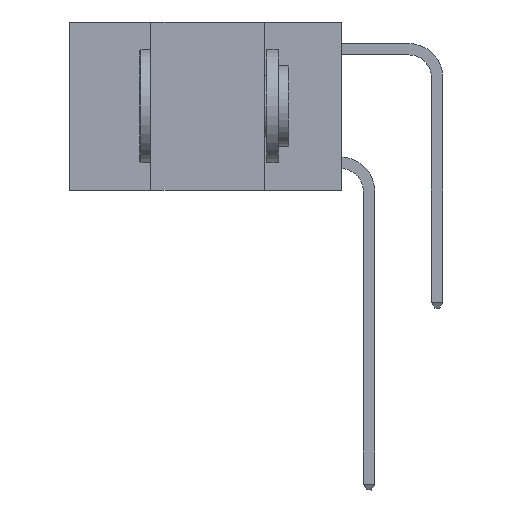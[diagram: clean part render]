
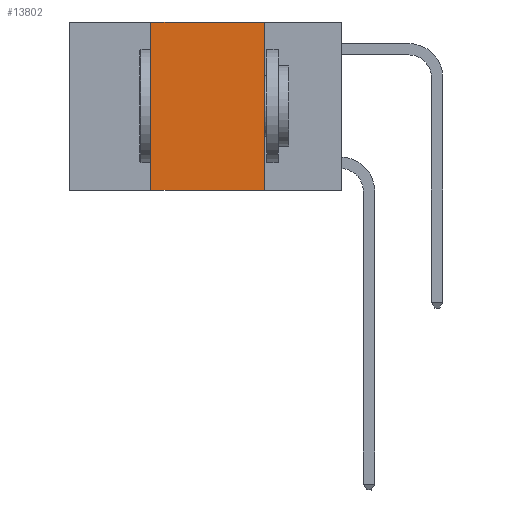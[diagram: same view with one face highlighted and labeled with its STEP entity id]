
A CAD part, left-side view. The second image highlights one B-rep face of the part: STEP entity #13802.
In plain terms, the highlighted planar face has unit normal (-1, 0, 0).
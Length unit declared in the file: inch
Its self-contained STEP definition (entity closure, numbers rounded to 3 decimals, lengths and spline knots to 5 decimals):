
#364 = CARTESIAN_POINT ( 'NONE',  ( 0., 0.6, 0. ) ) ;
#1477 = VECTOR ( 'NONE', #2226, 39.37008 ) ;
#1860 = DIRECTION ( 'NONE',  ( 1., 0., 0. ) ) ;
#2082 = LINE ( 'NONE', #364, #1477 ) ;
#2226 = DIRECTION ( 'NONE',  ( 0., -1., 0. ) ) ;
#3618 = VERTEX_POINT ( 'NONE', #18239 ) ;
#4120 = VERTEX_POINT ( 'NONE', #13554 ) ;
#4992 = CARTESIAN_POINT ( 'NONE',  ( 0., 0.42, 0. ) ) ;
#5948 = EDGE_CURVE ( 'NONE', #20587, #15449, #11277, .T. ) ;
#5998 = ORIENTED_EDGE ( 'NONE', *, *, #5948, .F. ) ;
#6011 = CARTESIAN_POINT ( 'NONE',  ( 0., 0.17, 0. ) ) ;
#6309 = ORIENTED_EDGE ( 'NONE', *, *, #12602, .F. ) ;
#6381 = ORIENTED_EDGE ( 'NONE', *, *, #20283, .F. ) ;
#6491 = ORIENTED_EDGE ( 'NONE', *, *, #10789, .T. ) ;
#7309 = PLANE ( 'NONE',  #18871 ) ;
#7601 = EDGE_LOOP ( 'NONE', ( #5998, #6309, #6381, #6491 ) ) ;
#8108 = CARTESIAN_POINT ( 'NONE',  ( 0., 0.17, -0.37 ) ) ;
#10789 = EDGE_CURVE ( 'NONE', #3618, #15449, #12400, .T. ) ;
#11277 = LINE ( 'NONE', #6011, #15445 ) ;
#12400 = LINE ( 'NONE', #20553, #15422 ) ;
#12602 = EDGE_CURVE ( 'NONE', #4120, #20587, #2082, .T. ) ;
#12739 = CARTESIAN_POINT ( 'NONE',  ( 0., 0.6, 0. ) ) ;
#13047 = VECTOR ( 'NONE', #17475, 39.37008 ) ;
#13554 = CARTESIAN_POINT ( 'NONE',  ( 0., 0.42, 0. ) ) ;
#13802 = ADVANCED_FACE ( 'NONE', ( #18910 ), #7309, .F. ) ;
#14503 = DIRECTION ( 'NONE',  ( 0., 0., -1. ) ) ;
#14766 = CARTESIAN_POINT ( 'NONE',  ( 0., 0.17, 0. ) ) ;
#15422 = VECTOR ( 'NONE', #22341, 39.37008 ) ;
#15445 = VECTOR ( 'NONE', #20267, 39.37008 ) ;
#15449 = VERTEX_POINT ( 'NONE', #8108 ) ;
#17475 = DIRECTION ( 'NONE',  ( 0., 0., 1. ) ) ;
#18239 = CARTESIAN_POINT ( 'NONE',  ( 0., 0.42, -0.37 ) ) ;
#18871 = AXIS2_PLACEMENT_3D ( 'NONE', #12739, #1860, #14503 ) ;
#18910 = FACE_OUTER_BOUND ( 'NONE', #7601, .T. ) ;
#20267 = DIRECTION ( 'NONE',  ( 0., 0., -1. ) ) ;
#20283 = EDGE_CURVE ( 'NONE', #3618, #4120, #22422, .T. ) ;
#20553 = CARTESIAN_POINT ( 'NONE',  ( 0., 0.6, -0.37 ) ) ;
#20587 = VERTEX_POINT ( 'NONE', #14766 ) ;
#22341 = DIRECTION ( 'NONE',  ( 0., -1., 0. ) ) ;
#22422 = LINE ( 'NONE', #4992, #13047 ) ;
